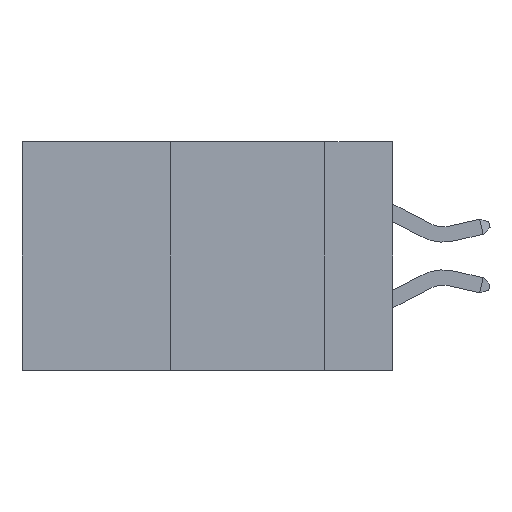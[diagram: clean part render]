
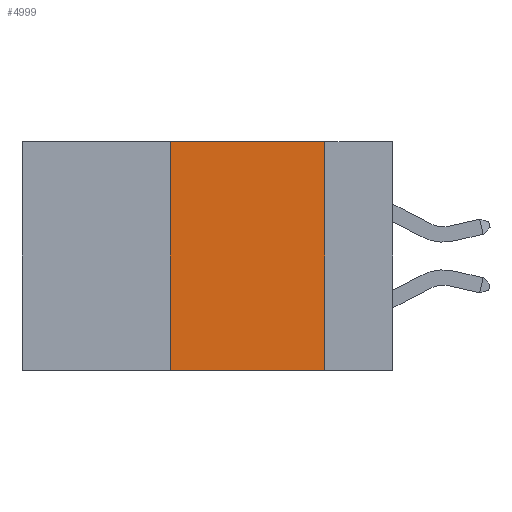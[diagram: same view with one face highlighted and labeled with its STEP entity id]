
A CAD part, left-side view. The second image highlights one B-rep face of the part: STEP entity #4999.
In plain terms, the highlighted planar face has unit normal (-1, 0, 0).
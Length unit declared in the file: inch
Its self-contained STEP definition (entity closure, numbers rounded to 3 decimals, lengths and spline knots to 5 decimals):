
#790 = DIRECTION ( 'NONE',  ( 0., 0., -1. ) ) ;
#1242 = PLANE ( 'NONE',  #25169 ) ;
#2183 = ORIENTED_EDGE ( 'NONE', *, *, #27126, .F. ) ;
#2231 = VERTEX_POINT ( 'NONE', #26648 ) ;
#4999 = ADVANCED_FACE ( 'NONE', ( #12967 ), #1242, .F. ) ;
#5178 = VERTEX_POINT ( 'NONE', #19271 ) ;
#5405 = VECTOR ( 'NONE', #13280, 39.37008 ) ;
#5577 = CARTESIAN_POINT ( 'NONE',  ( 0., 0.6, -0.37 ) ) ;
#6227 = EDGE_CURVE ( 'NONE', #7559, #5178, #23124, .T. ) ;
#6612 = CARTESIAN_POINT ( 'NONE',  ( 0., 0.11, 0. ) ) ;
#7559 = VERTEX_POINT ( 'NONE', #29856 ) ;
#7655 = CARTESIAN_POINT ( 'NONE',  ( 0., 0.6, 0. ) ) ;
#10647 = CARTESIAN_POINT ( 'NONE',  ( 0., 0.6, 0. ) ) ;
#11390 = ORIENTED_EDGE ( 'NONE', *, *, #28339, .F. ) ;
#12787 = VECTOR ( 'NONE', #16493, 39.37008 ) ;
#12967 = FACE_OUTER_BOUND ( 'NONE', #17974, .T. ) ;
#13280 = DIRECTION ( 'NONE',  ( 0., 0., 1. ) ) ;
#14018 = CARTESIAN_POINT ( 'NONE',  ( 0., 0.11, 0. ) ) ;
#16493 = DIRECTION ( 'NONE',  ( 0., -1., 0. ) ) ;
#17172 = EDGE_CURVE ( 'NONE', #7559, #2231, #24551, .T. ) ;
#17974 = EDGE_LOOP ( 'NONE', ( #11390, #2183, #18064, #25040 ) ) ;
#18064 = ORIENTED_EDGE ( 'NONE', *, *, #6227, .F. ) ;
#18500 = DIRECTION ( 'NONE',  ( 0., 0., -1. ) ) ;
#18949 = LINE ( 'NONE', #7655, #12787 ) ;
#19271 = CARTESIAN_POINT ( 'NONE',  ( 0., 0.36, 0. ) ) ;
#20064 = DIRECTION ( 'NONE',  ( 1., 0., 0. ) ) ;
#22943 = LINE ( 'NONE', #14018, #23154 ) ;
#23124 = LINE ( 'NONE', #27917, #5405 ) ;
#23154 = VECTOR ( 'NONE', #18500, 39.37008 ) ;
#23952 = VECTOR ( 'NONE', #29214, 39.37008 ) ;
#24551 = LINE ( 'NONE', #5577, #23952 ) ;
#25040 = ORIENTED_EDGE ( 'NONE', *, *, #17172, .T. ) ;
#25169 = AXIS2_PLACEMENT_3D ( 'NONE', #10647, #20064, #790 ) ;
#26458 = VERTEX_POINT ( 'NONE', #6612 ) ;
#26648 = CARTESIAN_POINT ( 'NONE',  ( 0., 0.11, -0.37 ) ) ;
#27126 = EDGE_CURVE ( 'NONE', #5178, #26458, #18949, .T. ) ;
#27917 = CARTESIAN_POINT ( 'NONE',  ( 0., 0.36, 0. ) ) ;
#28339 = EDGE_CURVE ( 'NONE', #26458, #2231, #22943, .T. ) ;
#29214 = DIRECTION ( 'NONE',  ( 0., -1., 0. ) ) ;
#29856 = CARTESIAN_POINT ( 'NONE',  ( 0., 0.36, -0.37 ) ) ;
